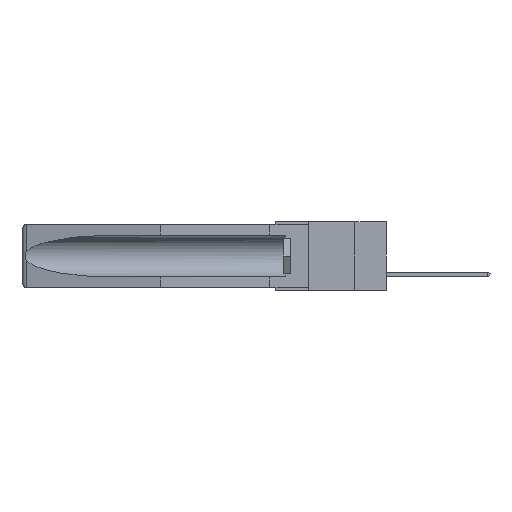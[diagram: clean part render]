
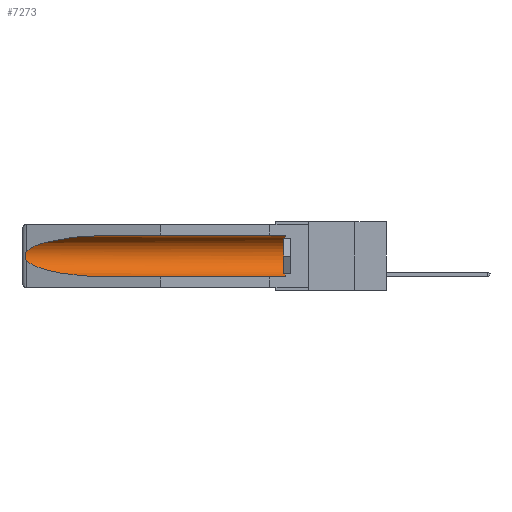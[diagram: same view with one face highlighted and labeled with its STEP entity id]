
A CAD part, left-side view. The second image highlights one B-rep face of the part: STEP entity #7273.
In plain terms, the highlighted cylindrical face has radius 2.857 mm (diameter 5.715 mm), a partial arc.
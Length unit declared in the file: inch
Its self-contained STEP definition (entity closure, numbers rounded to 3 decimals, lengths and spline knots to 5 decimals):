
#266 = CARTESIAN_POINT ( 'NONE',  ( 0.155, 0.126, -0.059 ) ) ;
#438 = CARTESIAN_POINT ( 'NONE',  ( 0.155, 0.126, -0.284 ) ) ;
#551 = CIRCLE ( 'NONE', #12942, 0.1125 ) ;
#603 = CARTESIAN_POINT ( 'NONE',  ( 0.26537, 1.52718, -0.19328 ) ) ;
#905 = EDGE_CURVE ( 'NONE', #14912, #7793, #2702, .T. ) ;
#962 = VERTEX_POINT ( 'NONE', #20787 ) ;
#1131 = CYLINDRICAL_SURFACE ( 'NONE', #19508, 0.1125 ) ;
#1464 = CARTESIAN_POINT ( 'NONE',  ( 0.21114, 1.30732, -0.059 ) ) ;
#1595 = ORIENTED_EDGE ( 'NONE', *, *, #905, .F. ) ;
#2039 = CARTESIAN_POINT ( 'NONE',  ( 0.155, 0.126, -0.1715 ) ) ;
#2346 = VERTEX_POINT ( 'NONE', #19440 ) ;
#2508 = CARTESIAN_POINT ( 'NONE',  ( 0.2673, 1.53269, -0.17917 ) ) ;
#2702 = LINE ( 'NONE', #7083, #4504 ) ;
#2717 = EDGE_CURVE ( 'NONE', #14912, #4881, #551, .T. ) ;
#3124 = EDGE_CURVE ( 'NONE', #4503, #7793, #11069, .T. ) ;
#3208 = CARTESIAN_POINT ( 'NONE',  ( 0.155, 1.07973, -0.059 ) ) ;
#3901 = CARTESIAN_POINT ( 'NONE',  ( 0.26537, 1.52718, -0.14972 ) ) ;
#4039 = CARTESIAN_POINT ( 'NONE',  ( 0.26597, 1.52961, -0.15275 ) ) ;
#4072 = EDGE_CURVE ( 'NONE', #2346, #4503, #13323, .T. ) ;
#4257 = EDGE_CURVE ( 'NONE', #962, #2346, #15311, .T. ) ;
#4503 = VERTEX_POINT ( 'NONE', #603 ) ;
#4504 = VECTOR ( 'NONE', #5612, 39.37008 ) ;
#4808 = CARTESIAN_POINT ( 'NONE',  ( 0.155, 1.07973, -0.284 ) ) ;
#4821 = CARTESIAN_POINT ( 'NONE',  ( 0.26537, 1.52718, -0.19328 ) ) ;
#4881 = VERTEX_POINT ( 'NONE', #266 ) ;
#5494 = CARTESIAN_POINT ( 'NONE',  ( 0.26654, 1.53092, -0.15636 ) ) ;
#5612 = DIRECTION ( 'NONE',  ( 0., 1., 0. ) ) ;
#5704 = CARTESIAN_POINT ( 'NONE',  ( 0.26597, 1.5296, -0.19026 ) ) ;
#5854 = CARTESIAN_POINT ( 'NONE',  ( 0.155, -0.30754, -0.059 ) ) ;
#6229 = DIRECTION ( 'NONE',  ( 0., 1., 0. ) ) ;
#6357 = CARTESIAN_POINT ( 'NONE',  ( 0.25451, 1.48313, -0.24835 ) ) ;
#7083 = CARTESIAN_POINT ( 'NONE',  ( 0.155, -0.30754, -0.284 ) ) ;
#7273 = ADVANCED_FACE ( 'NONE', ( #7667 ), #1131, .F. ) ;
#7327 = CARTESIAN_POINT ( 'NONE',  ( 0.26655, 1.53094, -0.18657 ) ) ;
#7667 = FACE_OUTER_BOUND ( 'NONE', #20449, .T. ) ;
#7793 = VERTEX_POINT ( 'NONE', #4808 ) ;
#8922 = CARTESIAN_POINT ( 'NONE',  ( 0.2675, 1.53308, -0.16763 ) ) ;
#9211 = DIRECTION ( 'NONE',  ( 0., 1., 0. ) ) ;
#10652 = ORIENTED_EDGE ( 'NONE', *, *, #4072, .T. ) ;
#10658 = CARTESIAN_POINT ( 'NONE',  ( 0.2675, 1.53308, -0.17534 ) ) ;
#11069 =( BOUNDED_CURVE ( )  B_SPLINE_CURVE ( 3, ( #4821, #6357, #14702, #15052 ),
 .UNSPECIFIED., .F., .F. ) 
 B_SPLINE_CURVE_WITH_KNOTS ( ( 4, 4 ),
 ( 0.1948, 1.5708 ),
 .UNSPECIFIED. ) 
 CURVE ( )  GEOMETRIC_REPRESENTATION_ITEM ( )  RATIONAL_B_SPLINE_CURVE ( ( 1., 0.848, 0.848, 1. ) ) 
 REPRESENTATION_ITEM ( '' )  );
#12069 = DIRECTION ( 'NONE',  ( 0., 0., 1. ) ) ;
#12244 = ORIENTED_EDGE ( 'NONE', *, *, #18349, .T. ) ;
#12933 = CARTESIAN_POINT ( 'NONE',  ( 0.26537, 1.52718, -0.14972 ) ) ;
#12942 = AXIS2_PLACEMENT_3D ( 'NONE', #2039, #18648, #12069 ) ;
#13323 = B_SPLINE_CURVE_WITH_KNOTS ( 'NONE', 3,
 ( #3901, #4039, #5494, #15631, #8922, #10658, #2508, #7327, #5704, #18840 ),
 .UNSPECIFIED., .F., .F.,
 ( 4, 2, 2, 2, 4 ),
 ( 0., 0.00029, 0.00058, 0.00087, 0.00117 ),
 .UNSPECIFIED. ) ;
#14497 = CARTESIAN_POINT ( 'NONE',  ( 0.155, -0.30754, -0.1715 ) ) ;
#14702 = CARTESIAN_POINT ( 'NONE',  ( 0.21114, 1.30732, -0.284 ) ) ;
#14912 = VERTEX_POINT ( 'NONE', #438 ) ;
#15052 = CARTESIAN_POINT ( 'NONE',  ( 0.155, 1.07973, -0.284 ) ) ;
#15311 =( BOUNDED_CURVE ( )  B_SPLINE_CURVE ( 3, ( #3208, #1464, #18064, #12933 ),
 .UNSPECIFIED., .F., .F. ) 
 B_SPLINE_CURVE_WITH_KNOTS ( ( 4, 4 ),
 ( 4.71239, 6.08839 ),
 .UNSPECIFIED. ) 
 CURVE ( )  GEOMETRIC_REPRESENTATION_ITEM ( )  RATIONAL_B_SPLINE_CURVE ( ( 1., 0.848, 0.848, 1. ) ) 
 REPRESENTATION_ITEM ( '' )  );
#15631 = CARTESIAN_POINT ( 'NONE',  ( 0.2673, 1.5327, -0.16383 ) ) ;
#16963 = ORIENTED_EDGE ( 'NONE', *, *, #2717, .T. ) ;
#17464 = LINE ( 'NONE', #5854, #20873 ) ;
#17833 = DIRECTION ( 'NONE',  ( 0., 0., 1. ) ) ;
#18064 = CARTESIAN_POINT ( 'NONE',  ( 0.25451, 1.48313, -0.09465 ) ) ;
#18349 = EDGE_CURVE ( 'NONE', #4881, #962, #17464, .T. ) ;
#18648 = DIRECTION ( 'NONE',  ( 0., -1., 0. ) ) ;
#18840 = CARTESIAN_POINT ( 'NONE',  ( 0.26537, 1.52718, -0.19328 ) ) ;
#19440 = CARTESIAN_POINT ( 'NONE',  ( 0.26537, 1.52718, -0.14972 ) ) ;
#19508 = AXIS2_PLACEMENT_3D ( 'NONE', #14497, #6229, #17833 ) ;
#20449 = EDGE_LOOP ( 'NONE', ( #20649, #10652, #20754, #1595, #16963, #12244 ) ) ;
#20649 = ORIENTED_EDGE ( 'NONE', *, *, #4257, .T. ) ;
#20754 = ORIENTED_EDGE ( 'NONE', *, *, #3124, .T. ) ;
#20787 = CARTESIAN_POINT ( 'NONE',  ( 0.155, 1.07973, -0.059 ) ) ;
#20873 = VECTOR ( 'NONE', #9211, 39.37008 ) ;
